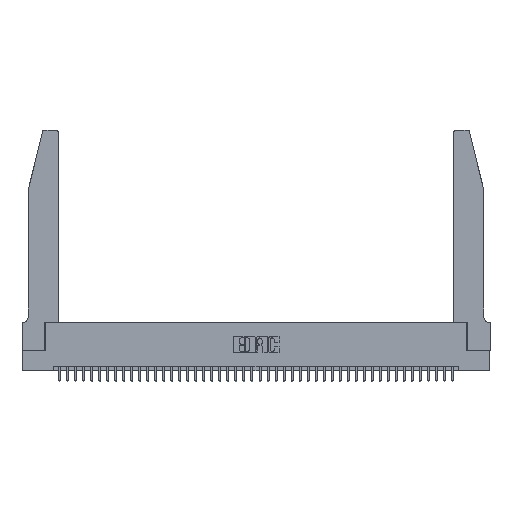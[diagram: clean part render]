
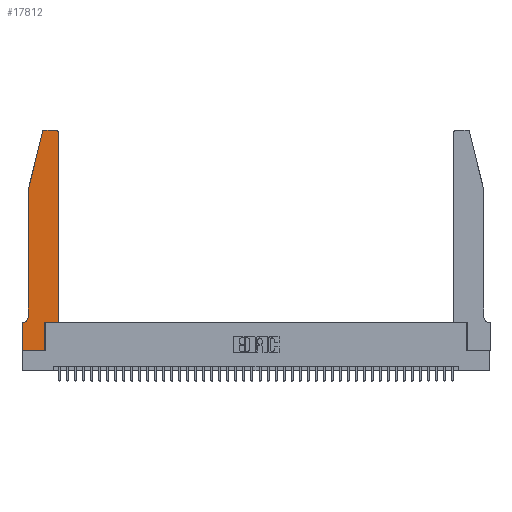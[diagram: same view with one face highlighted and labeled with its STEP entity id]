
A CAD part, top view. The second image highlights one B-rep face of the part: STEP entity #17812.
In plain terms, the highlighted planar face has unit normal (0, 0, 1).
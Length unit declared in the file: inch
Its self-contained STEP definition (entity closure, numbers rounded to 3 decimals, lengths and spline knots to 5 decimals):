
#248 = VECTOR ( 'NONE', #15388, 39.37008 ) ;
#1436 = LINE ( 'NONE', #25899, #29512 ) ;
#1590 = VERTEX_POINT ( 'NONE', #8602 ) ;
#1948 = LINE ( 'NONE', #17059, #39296 ) ;
#2122 = CARTESIAN_POINT ( 'NONE',  ( 0.0755, 0.35, 0.37 ) ) ;
#3499 = DIRECTION ( 'NONE',  ( -0.239, -0.971, 0. ) ) ;
#5093 = CIRCLE ( 'NONE', #35365, 0.03 ) ;
#5116 = FACE_OUTER_BOUND ( 'NONE', #7085, .T. ) ;
#5450 = DIRECTION ( 'NONE',  ( -1., 0., 0. ) ) ;
#5619 = EDGE_CURVE ( 'NONE', #13587, #33600, #32636, .T. ) ;
#6183 = ORIENTED_EDGE ( 'NONE', *, *, #35713, .T. ) ;
#6362 = DIRECTION ( 'NONE',  ( 0., 0., 1. ) ) ;
#6614 = DIRECTION ( 'NONE',  ( -1., 0., 0. ) ) ;
#6636 = AXIS2_PLACEMENT_3D ( 'NONE', #28710, #32036, #15486 ) ;
#7085 = EDGE_LOOP ( 'NONE', ( #16075, #6183, #28381, #22318, #39357, #36428, #21137, #18540, #8536, #8902, #32208, #10570 ) ) ;
#8193 = VERTEX_POINT ( 'NONE', #39629 ) ;
#8536 = ORIENTED_EDGE ( 'NONE', *, *, #12393, .T. ) ;
#8546 = DIRECTION ( 'NONE',  ( 1., 0., 0. ) ) ;
#8573 = DIRECTION ( 'NONE',  ( 0., -1., 0. ) ) ;
#8602 = CARTESIAN_POINT ( 'NONE',  ( 0.4505, 0.35, 0.37 ) ) ;
#8902 = ORIENTED_EDGE ( 'NONE', *, *, #18877, .T. ) ;
#9323 = CARTESIAN_POINT ( 'NONE',  ( 0.4205, 2.72, 0.37 ) ) ;
#10433 = AXIS2_PLACEMENT_3D ( 'NONE', #21388, #28108, #20803 ) ;
#10570 = ORIENTED_EDGE ( 'NONE', *, *, #18216, .T. ) ;
#11060 = VERTEX_POINT ( 'NONE', #16299 ) ;
#11618 = CARTESIAN_POINT ( 'NONE',  ( 0., 0., 0.37 ) ) ;
#12393 = EDGE_CURVE ( 'NONE', #21130, #8193, #1948, .T. ) ;
#12616 = DIRECTION ( 'NONE',  ( 1., 0., 0. ) ) ;
#12796 = VECTOR ( 'NONE', #16194, 39.37008 ) ;
#13205 = PLANE ( 'NONE',  #26657 ) ;
#13472 = VERTEX_POINT ( 'NONE', #22087 ) ;
#13587 = VERTEX_POINT ( 'NONE', #22323 ) ;
#14876 = LINE ( 'NONE', #2122, #29441 ) ;
#15388 = DIRECTION ( 'NONE',  ( 0., -1., 0. ) ) ;
#15486 = DIRECTION ( 'NONE',  ( -1., 0., 0. ) ) ;
#15919 = LINE ( 'NONE', #25637, #12796 ) ;
#16075 = ORIENTED_EDGE ( 'NONE', *, *, #29167, .T. ) ;
#16194 = DIRECTION ( 'NONE',  ( 1., 0., 0. ) ) ;
#16299 = CARTESIAN_POINT ( 'NONE',  ( 0.0055, 0.35, 0.37 ) ) ;
#16587 = CARTESIAN_POINT ( 'NONE',  ( 0.0755, 0.42, 0.37 ) ) ;
#16859 = VERTEX_POINT ( 'NONE', #36470 ) ;
#16899 = EDGE_CURVE ( 'NONE', #25793, #11060, #21741, .T. ) ;
#17059 = CARTESIAN_POINT ( 'NONE',  ( 0.2865, 0.35, 0.37 ) ) ;
#17416 = CARTESIAN_POINT ( 'NONE',  ( 0.284, 2.75, 0.37 ) ) ;
#17812 = ADVANCED_FACE ( 'NONE', ( #5116 ), #13205, .T. ) ;
#18100 = VECTOR ( 'NONE', #3499, 39.37008 ) ;
#18216 = EDGE_CURVE ( 'NONE', #13472, #16859, #5093, .T. ) ;
#18540 = ORIENTED_EDGE ( 'NONE', *, *, #30575, .T. ) ;
#18877 = EDGE_CURVE ( 'NONE', #8193, #1590, #15919, .T. ) ;
#19640 = EDGE_CURVE ( 'NONE', #33600, #25793, #27810, .T. ) ;
#20033 = VERTEX_POINT ( 'NONE', #31964 ) ;
#20284 = LINE ( 'NONE', #28439, #24383 ) ;
#20417 = CARTESIAN_POINT ( 'NONE',  ( 0.0755, 2., 0.37 ) ) ;
#20547 = DIRECTION ( 'NONE',  ( 0., 1., 0. ) ) ;
#20803 = DIRECTION ( 'NONE',  ( 1., 0., 0. ) ) ;
#21130 = VERTEX_POINT ( 'NONE', #30664 ) ;
#21137 = ORIENTED_EDGE ( 'NONE', *, *, #37964, .T. ) ;
#21388 = CARTESIAN_POINT ( 'NONE',  ( 0.284, 2.72, 0.37 ) ) ;
#21741 = CIRCLE ( 'NONE', #6636, 0.07 ) ;
#22087 = CARTESIAN_POINT ( 'NONE',  ( 0.4505, 2.72, 0.37 ) ) ;
#22318 = ORIENTED_EDGE ( 'NONE', *, *, #19640, .T. ) ;
#22323 = CARTESIAN_POINT ( 'NONE',  ( 0.25487, 2.72718, 0.37 ) ) ;
#23508 = LINE ( 'NONE', #11618, #29829 ) ;
#24383 = VECTOR ( 'NONE', #8546, 39.37008 ) ;
#25575 = EDGE_CURVE ( 'NONE', #1590, #13472, #1436, .T. ) ;
#25637 = CARTESIAN_POINT ( 'NONE',  ( 0.4505, 0.35, 0.37 ) ) ;
#25793 = VERTEX_POINT ( 'NONE', #16587 ) ;
#25833 = VERTEX_POINT ( 'NONE', #17416 ) ;
#25899 = CARTESIAN_POINT ( 'NONE',  ( 0.4505, 0.35, 0.37 ) ) ;
#26657 = AXIS2_PLACEMENT_3D ( 'NONE', #36369, #6362, #12616 ) ;
#27810 = LINE ( 'NONE', #28624, #248 ) ;
#28108 = DIRECTION ( 'NONE',  ( 0., 0., 1. ) ) ;
#28381 = ORIENTED_EDGE ( 'NONE', *, *, #5619, .T. ) ;
#28439 = CARTESIAN_POINT ( 'NONE',  ( 0., 0., 0.37 ) ) ;
#28624 = CARTESIAN_POINT ( 'NONE',  ( 0.0755, 2., 0.37 ) ) ;
#28643 = LINE ( 'NONE', #30014, #33778 ) ;
#28710 = CARTESIAN_POINT ( 'NONE',  ( 0.0055, 0.42, 0.37 ) ) ;
#29167 = EDGE_CURVE ( 'NONE', #16859, #25833, #28643, .T. ) ;
#29265 = DIRECTION ( 'NONE',  ( 0., 1., 0. ) ) ;
#29346 = DIRECTION ( 'NONE',  ( 1., 0., 0. ) ) ;
#29441 = VECTOR ( 'NONE', #5450, 39.37008 ) ;
#29512 = VECTOR ( 'NONE', #29265, 39.37008 ) ;
#29829 = VECTOR ( 'NONE', #8573, 39.37008 ) ;
#30014 = CARTESIAN_POINT ( 'NONE',  ( 0.2605, 2.75, 0.37 ) ) ;
#30575 = EDGE_CURVE ( 'NONE', #20033, #21130, #20284, .T. ) ;
#30664 = CARTESIAN_POINT ( 'NONE',  ( 0.2865, 0., 0.37 ) ) ;
#31964 = CARTESIAN_POINT ( 'NONE',  ( 0., 0., 0.37 ) ) ;
#32036 = DIRECTION ( 'NONE',  ( 0., 0., -1. ) ) ;
#32208 = ORIENTED_EDGE ( 'NONE', *, *, #25575, .T. ) ;
#32636 = LINE ( 'NONE', #20417, #18100 ) ;
#33127 = VERTEX_POINT ( 'NONE', #38599 ) ;
#33600 = VERTEX_POINT ( 'NONE', #34480 ) ;
#33778 = VECTOR ( 'NONE', #6614, 39.37008 ) ;
#34433 = EDGE_CURVE ( 'NONE', #11060, #33127, #14876, .T. ) ;
#34480 = CARTESIAN_POINT ( 'NONE',  ( 0.0755, 2., 0.37 ) ) ;
#35365 = AXIS2_PLACEMENT_3D ( 'NONE', #9323, #42505, #29346 ) ;
#35713 = EDGE_CURVE ( 'NONE', #25833, #13587, #40225, .T. ) ;
#36369 = CARTESIAN_POINT ( 'NONE',  ( 0., 0.35, 0.37 ) ) ;
#36428 = ORIENTED_EDGE ( 'NONE', *, *, #34433, .T. ) ;
#36470 = CARTESIAN_POINT ( 'NONE',  ( 0.4205, 2.75, 0.37 ) ) ;
#37964 = EDGE_CURVE ( 'NONE', #33127, #20033, #23508, .T. ) ;
#38599 = CARTESIAN_POINT ( 'NONE',  ( 0., 0.35, 0.37 ) ) ;
#39296 = VECTOR ( 'NONE', #20547, 39.37008 ) ;
#39357 = ORIENTED_EDGE ( 'NONE', *, *, #16899, .T. ) ;
#39629 = CARTESIAN_POINT ( 'NONE',  ( 0.2865, 0.35, 0.37 ) ) ;
#40225 = CIRCLE ( 'NONE', #10433, 0.03 ) ;
#42505 = DIRECTION ( 'NONE',  ( 0., 0., 1. ) ) ;
